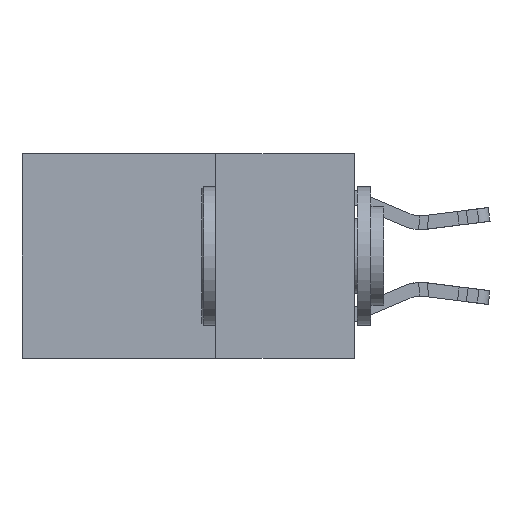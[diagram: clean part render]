
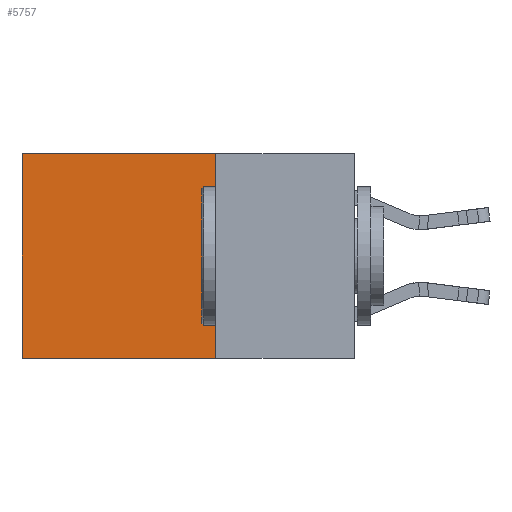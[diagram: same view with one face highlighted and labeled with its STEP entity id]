
A CAD part, left-side view. The second image highlights one B-rep face of the part: STEP entity #5757.
In plain terms, the highlighted planar face has unit normal (-1, 0, 0).
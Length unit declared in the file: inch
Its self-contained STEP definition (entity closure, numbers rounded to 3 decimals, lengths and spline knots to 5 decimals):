
#1116 = LINE ( 'NONE', #8423, #26678 ) ;
#1491 = VECTOR ( 'NONE', #13243, 39.37008 ) ;
#2923 = CARTESIAN_POINT ( 'NONE',  ( 0.2625, 0.25, 0. ) ) ;
#3701 = FACE_OUTER_BOUND ( 'NONE', #23850, .T. ) ;
#4467 = EDGE_CURVE ( 'NONE', #11341, #15872, #6717, .T. ) ;
#4992 = LINE ( 'NONE', #2923, #6729 ) ;
#5000 = VERTEX_POINT ( 'NONE', #23877 ) ;
#5757 = ADVANCED_FACE ( 'NONE', ( #3701 ), #8636, .F. ) ;
#5775 = ORIENTED_EDGE ( 'NONE', *, *, #4467, .T. ) ;
#6717 = LINE ( 'NONE', #28369, #11484 ) ;
#6729 = VECTOR ( 'NONE', #12650, 39.37008 ) ;
#8423 = CARTESIAN_POINT ( 'NONE',  ( 0.2625, 0.25, 0. ) ) ;
#8636 = PLANE ( 'NONE',  #15301 ) ;
#10598 = VERTEX_POINT ( 'NONE', #29226 ) ;
#11341 = VERTEX_POINT ( 'NONE', #30795 ) ;
#11484 = VECTOR ( 'NONE', #16290, 39.37008 ) ;
#12316 = ORIENTED_EDGE ( 'NONE', *, *, #21327, .F. ) ;
#12650 = DIRECTION ( 'NONE',  ( 0., 0., -1. ) ) ;
#13243 = DIRECTION ( 'NONE',  ( 0., 1., 0. ) ) ;
#14540 = ORIENTED_EDGE ( 'NONE', *, *, #29515, .T. ) ;
#15301 = AXIS2_PLACEMENT_3D ( 'NONE', #18367, #28057, #25682 ) ;
#15872 = VERTEX_POINT ( 'NONE', #27550 ) ;
#16290 = DIRECTION ( 'NONE',  ( 0., 0., -1. ) ) ;
#18367 = CARTESIAN_POINT ( 'NONE',  ( 0.2625, 0.25, 0. ) ) ;
#21327 = EDGE_CURVE ( 'NONE', #10598, #15872, #22490, .T. ) ;
#22490 = LINE ( 'NONE', #27708, #1491 ) ;
#23082 = DIRECTION ( 'NONE',  ( 0., 1., 0. ) ) ;
#23850 = EDGE_LOOP ( 'NONE', ( #5775, #12316, #26510, #14540 ) ) ;
#23877 = CARTESIAN_POINT ( 'NONE',  ( 0.2625, 0.25, 0. ) ) ;
#25055 = EDGE_CURVE ( 'NONE', #5000, #10598, #4992, .T. ) ;
#25682 = DIRECTION ( 'NONE',  ( 0., 0., -1. ) ) ;
#26510 = ORIENTED_EDGE ( 'NONE', *, *, #25055, .F. ) ;
#26678 = VECTOR ( 'NONE', #23082, 39.37008 ) ;
#27550 = CARTESIAN_POINT ( 'NONE',  ( 0.2625, 0.6, -0.37 ) ) ;
#27708 = CARTESIAN_POINT ( 'NONE',  ( 0.2625, 0.25, -0.37 ) ) ;
#28057 = DIRECTION ( 'NONE',  ( 1., 0., 0. ) ) ;
#28369 = CARTESIAN_POINT ( 'NONE',  ( 0.2625, 0.6, 0. ) ) ;
#29226 = CARTESIAN_POINT ( 'NONE',  ( 0.2625, 0.25, -0.37 ) ) ;
#29515 = EDGE_CURVE ( 'NONE', #5000, #11341, #1116, .T. ) ;
#30795 = CARTESIAN_POINT ( 'NONE',  ( 0.2625, 0.6, 0. ) ) ;
